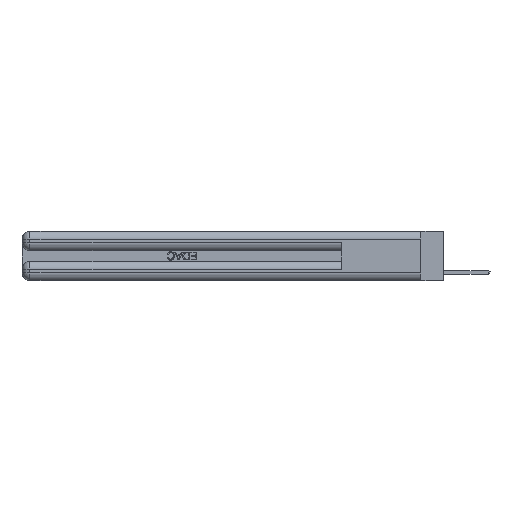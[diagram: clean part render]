
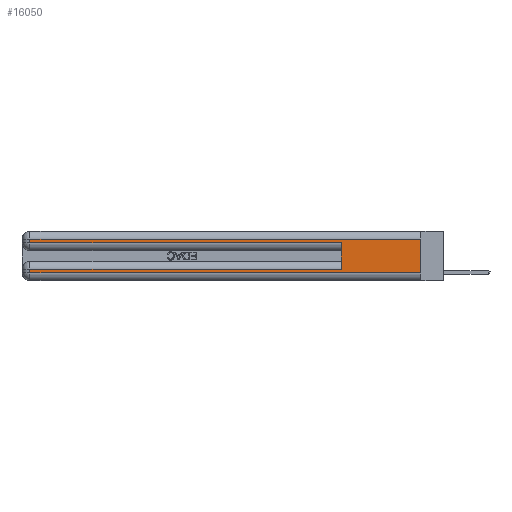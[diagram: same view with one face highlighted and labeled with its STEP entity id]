
A CAD part, left-side view. The second image highlights one B-rep face of the part: STEP entity #16050.
In plain terms, the highlighted planar face has unit normal (-1, 0, 0).
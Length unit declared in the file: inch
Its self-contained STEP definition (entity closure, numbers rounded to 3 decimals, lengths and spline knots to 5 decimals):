
#76 = CARTESIAN_POINT ( 'NONE',  ( 0., 0., 0.06 ) ) ;
#679 = VERTEX_POINT ( 'NONE', #17571 ) ;
#1555 = LINE ( 'NONE', #3860, #8923 ) ;
#1757 = CARTESIAN_POINT ( 'NONE',  ( 0., 2.94, 0.37 ) ) ;
#2030 = AXIS2_PLACEMENT_3D ( 'NONE', #19953, #4472, #22192 ) ;
#2840 = EDGE_LOOP ( 'NONE', ( #25169, #12063, #7537, #23465, #15251, #8429, #18134, #9640 ) ) ;
#3003 = CARTESIAN_POINT ( 'NONE',  ( 0., 2.94, 0.085 ) ) ;
#3105 = EDGE_CURVE ( 'NONE', #679, #6224, #9501, .T. ) ;
#3648 = VECTOR ( 'NONE', #20898, 39.37008 ) ;
#3860 = CARTESIAN_POINT ( 'NONE',  ( 0., 0., 0.31 ) ) ;
#4431 = LINE ( 'NONE', #1757, #6159 ) ;
#4472 = DIRECTION ( 'NONE',  ( 1., 0., 0. ) ) ;
#4762 = DIRECTION ( 'NONE',  ( 0., 0., -1. ) ) ;
#6159 = VECTOR ( 'NONE', #22112, 39.37008 ) ;
#6224 = VERTEX_POINT ( 'NONE', #76 ) ;
#6619 = DIRECTION ( 'NONE',  ( 0., -1., 0. ) ) ;
#6777 = LINE ( 'NONE', #7685, #3648 ) ;
#6827 = VECTOR ( 'NONE', #4762, 39.37008 ) ;
#6997 = VERTEX_POINT ( 'NONE', #27434 ) ;
#7537 = ORIENTED_EDGE ( 'NONE', *, *, #9538, .T. ) ;
#7685 = CARTESIAN_POINT ( 'NONE',  ( 0., 0.6, 0.145 ) ) ;
#8429 = ORIENTED_EDGE ( 'NONE', *, *, #21920, .T. ) ;
#8923 = VECTOR ( 'NONE', #28264, 39.37008 ) ;
#9501 = LINE ( 'NONE', #26254, #19250 ) ;
#9538 = EDGE_CURVE ( 'NONE', #16680, #24665, #22521, .T. ) ;
#9600 = DIRECTION ( 'NONE',  ( 0., 1., 0. ) ) ;
#9618 = VERTEX_POINT ( 'NONE', #3003 ) ;
#9640 = ORIENTED_EDGE ( 'NONE', *, *, #3105, .T. ) ;
#9771 = EDGE_CURVE ( 'NONE', #6997, #6224, #26689, .T. ) ;
#9871 = EDGE_CURVE ( 'NONE', #6997, #16680, #1555, .T. ) ;
#10176 = FACE_OUTER_BOUND ( 'NONE', #2840, .T. ) ;
#12063 = ORIENTED_EDGE ( 'NONE', *, *, #9871, .T. ) ;
#12337 = VECTOR ( 'NONE', #9600, 39.37008 ) ;
#13586 = CARTESIAN_POINT ( 'NONE',  ( 0., 0., 0.085 ) ) ;
#13609 = EDGE_CURVE ( 'NONE', #25616, #20765, #6777, .T. ) ;
#15128 = DIRECTION ( 'NONE',  ( 0., -1., 0. ) ) ;
#15251 = ORIENTED_EDGE ( 'NONE', *, *, #13609, .F. ) ;
#15488 = CARTESIAN_POINT ( 'NONE',  ( 0., 0.6, 0.285 ) ) ;
#15943 = CARTESIAN_POINT ( 'NONE',  ( 0., 0., 0.285 ) ) ;
#16050 = ADVANCED_FACE ( 'NONE', ( #10176 ), #28475, .F. ) ;
#16341 = CARTESIAN_POINT ( 'NONE',  ( 0., 2.94, 0.31 ) ) ;
#16680 = VERTEX_POINT ( 'NONE', #16341 ) ;
#16918 = VECTOR ( 'NONE', #21295, 39.37008 ) ;
#17571 = CARTESIAN_POINT ( 'NONE',  ( 0., 2.94, 0.06 ) ) ;
#18134 = ORIENTED_EDGE ( 'NONE', *, *, #20518, .T. ) ;
#18299 = LINE ( 'NONE', #13586, #12337 ) ;
#19250 = VECTOR ( 'NONE', #15128, 39.37008 ) ;
#19454 = CARTESIAN_POINT ( 'NONE',  ( 0., 2.94, 0.285 ) ) ;
#19953 = CARTESIAN_POINT ( 'NONE',  ( 0., 0., 0.37 ) ) ;
#20495 = VECTOR ( 'NONE', #6619, 39.37008 ) ;
#20518 = EDGE_CURVE ( 'NONE', #9618, #679, #4431, .T. ) ;
#20765 = VERTEX_POINT ( 'NONE', #15488 ) ;
#20898 = DIRECTION ( 'NONE',  ( 0., 0., 1. ) ) ;
#21295 = DIRECTION ( 'NONE',  ( 0., 0., -1. ) ) ;
#21920 = EDGE_CURVE ( 'NONE', #25616, #9618, #18299, .T. ) ;
#22112 = DIRECTION ( 'NONE',  ( 0., 0., -1. ) ) ;
#22192 = DIRECTION ( 'NONE',  ( 0., 0., -1. ) ) ;
#22521 = LINE ( 'NONE', #28967, #6827 ) ;
#23277 = CARTESIAN_POINT ( 'NONE',  ( 0., 0., 0.37 ) ) ;
#23465 = ORIENTED_EDGE ( 'NONE', *, *, #25946, .T. ) ;
#24665 = VERTEX_POINT ( 'NONE', #19454 ) ;
#25169 = ORIENTED_EDGE ( 'NONE', *, *, #9771, .F. ) ;
#25480 = CARTESIAN_POINT ( 'NONE',  ( 0., 0.6, 0.085 ) ) ;
#25616 = VERTEX_POINT ( 'NONE', #25480 ) ;
#25946 = EDGE_CURVE ( 'NONE', #24665, #20765, #28562, .T. ) ;
#26254 = CARTESIAN_POINT ( 'NONE',  ( 0., 0., 0.06 ) ) ;
#26689 = LINE ( 'NONE', #23277, #16918 ) ;
#27434 = CARTESIAN_POINT ( 'NONE',  ( 0., 0., 0.31 ) ) ;
#28264 = DIRECTION ( 'NONE',  ( 0., 1., 0. ) ) ;
#28475 = PLANE ( 'NONE',  #2030 ) ;
#28562 = LINE ( 'NONE', #15943, #20495 ) ;
#28967 = CARTESIAN_POINT ( 'NONE',  ( 0., 2.94, 0.37 ) ) ;
